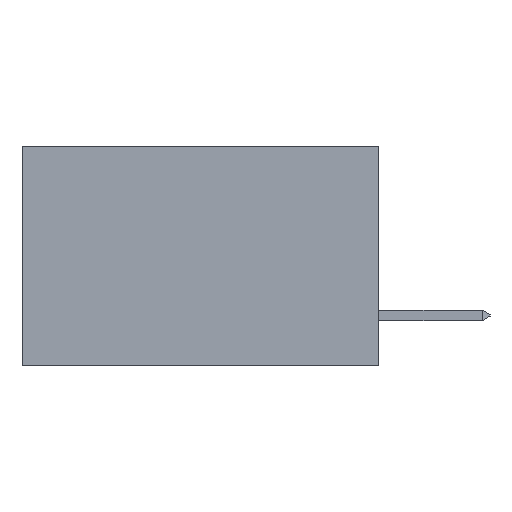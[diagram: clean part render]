
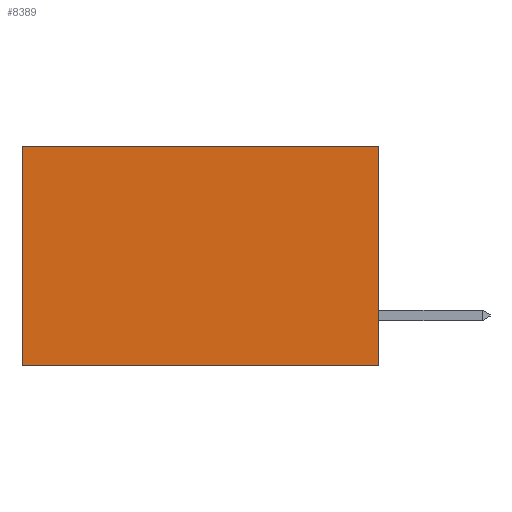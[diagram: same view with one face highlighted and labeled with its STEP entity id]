
A CAD part, left-side view. The second image highlights one B-rep face of the part: STEP entity #8389.
In plain terms, the highlighted planar face has unit normal (-1, 0, 0).
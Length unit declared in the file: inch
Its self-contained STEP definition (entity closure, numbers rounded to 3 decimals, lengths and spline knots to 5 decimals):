
#281 = EDGE_CURVE ( 'NONE', #17100, #15209, #11776, .T. ) ;
#730 = ORIENTED_EDGE ( 'NONE', *, *, #281, .T. ) ;
#2122 = VECTOR ( 'NONE', #15146, 39.37008 ) ;
#2840 = DIRECTION ( 'NONE',  ( 0., 0., -1. ) ) ;
#3146 = EDGE_CURVE ( 'NONE', #14777, #17100, #13630, .T. ) ;
#3616 = EDGE_LOOP ( 'NONE', ( #730, #7371, #8713, #7723 ) ) ;
#3902 = LINE ( 'NONE', #4275, #7325 ) ;
#4272 = DIRECTION ( 'NONE',  ( 0., 0., -1. ) ) ;
#4275 = CARTESIAN_POINT ( 'NONE',  ( 0.298, 0., 0. ) ) ;
#4910 = CARTESIAN_POINT ( 'NONE',  ( 0.298, 0., -0.37 ) ) ;
#6108 = EDGE_CURVE ( 'NONE', #14777, #12554, #3902, .T. ) ;
#6204 = CARTESIAN_POINT ( 'NONE',  ( 0.298, 0., -0.37 ) ) ;
#6627 = DIRECTION ( 'NONE',  ( 0., 1., 0. ) ) ;
#7325 = VECTOR ( 'NONE', #4272, 39.37008 ) ;
#7371 = ORIENTED_EDGE ( 'NONE', *, *, #15155, .F. ) ;
#7723 = ORIENTED_EDGE ( 'NONE', *, *, #3146, .T. ) ;
#8041 = CARTESIAN_POINT ( 'NONE',  ( 0.298, 0.6, 0. ) ) ;
#8389 = ADVANCED_FACE ( 'NONE', ( #10516 ), #10787, .F. ) ;
#8713 = ORIENTED_EDGE ( 'NONE', *, *, #6108, .F. ) ;
#10516 = FACE_OUTER_BOUND ( 'NONE', #3616, .T. ) ;
#10787 = PLANE ( 'NONE',  #16930 ) ;
#10808 = CARTESIAN_POINT ( 'NONE',  ( 0.298, 0., 0. ) ) ;
#10810 = DIRECTION ( 'NONE',  ( 1., 0., 0. ) ) ;
#10828 = DIRECTION ( 'NONE',  ( 0., 0., -1. ) ) ;
#11254 = VECTOR ( 'NONE', #2840, 39.37008 ) ;
#11632 = CARTESIAN_POINT ( 'NONE',  ( 0.298, 0.6, -0.37 ) ) ;
#11651 = VECTOR ( 'NONE', #6627, 39.37008 ) ;
#11776 = LINE ( 'NONE', #8041, #11254 ) ;
#12554 = VERTEX_POINT ( 'NONE', #6204 ) ;
#13523 = CARTESIAN_POINT ( 'NONE',  ( 0.298, 0., 0. ) ) ;
#13630 = LINE ( 'NONE', #14553, #2122 ) ;
#14553 = CARTESIAN_POINT ( 'NONE',  ( 0.298, 0., 0. ) ) ;
#14777 = VERTEX_POINT ( 'NONE', #13523 ) ;
#15146 = DIRECTION ( 'NONE',  ( 0., 1., 0. ) ) ;
#15155 = EDGE_CURVE ( 'NONE', #12554, #15209, #19857, .T. ) ;
#15209 = VERTEX_POINT ( 'NONE', #11632 ) ;
#16469 = CARTESIAN_POINT ( 'NONE',  ( 0.298, 0.6, 0. ) ) ;
#16930 = AXIS2_PLACEMENT_3D ( 'NONE', #10808, #10810, #10828 ) ;
#17100 = VERTEX_POINT ( 'NONE', #16469 ) ;
#19857 = LINE ( 'NONE', #4910, #11651 ) ;
